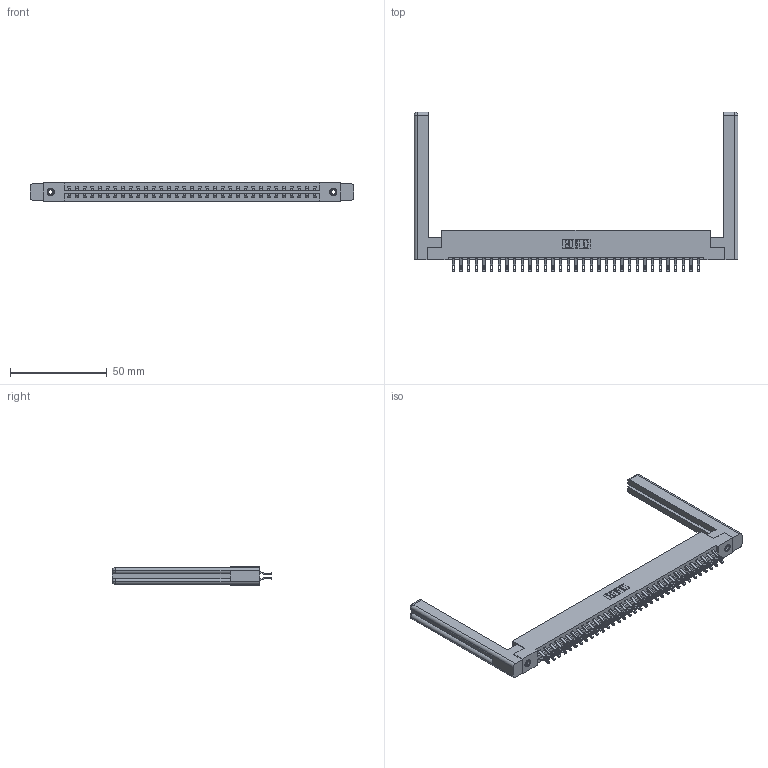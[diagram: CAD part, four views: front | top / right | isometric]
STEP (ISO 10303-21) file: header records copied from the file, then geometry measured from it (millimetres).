
FILE_DESCRIPTION (( 'STEP AP203' ), '1' );
FILE_NAME ('387-066-555-258.STEP', '2019-10-19T19:16:40', ( '' ), ( '' ), 'SwSTEP 2.0', 'SolidWorks 2016', '' );
FILE_SCHEMA (( 'CONFIG_CONTROL_DESIGN' ));
Length unit declared in the file: inch
Products named in the file (5): 337 Part_Flush Mounting Lugs - 0.156 Dia-TI; 345-292-001_555 Tail; 345-250-001_345-250-001-102; 307-220-058; 387-066-555-258
Assembly tree (71 placements, depth 2):
  387-066-555-258
    337 Part_Flush Mounting Lugs - 0.156 Dia-TI
    345-292-001_555 Tail  x66
    345-250-001_345-250-001-102  x2
    307-220-058  x2
Bounding box: 167.39 x 82.56 x 9.4 mm (x, y, z)
Volume: 24854.4 mm3; surface area: 25704.3 mm2
Topology: 71 solids, 71 shells, 4216 faces, 13139 edges, 8746 vertices
Faces by surface type: plane 2530, cylinder 1662, cone 12, torus 12
Entity records: 29710 total; most frequent: CARTESIAN_POINT 5055, ORIENTED_EDGE 4900, DIRECTION 4302, EDGE_CURVE 2450, VECTOR 2254, LINE 2254, VERTEX_POINT 1626, AXIS2_PLACEMENT_3D 1024
